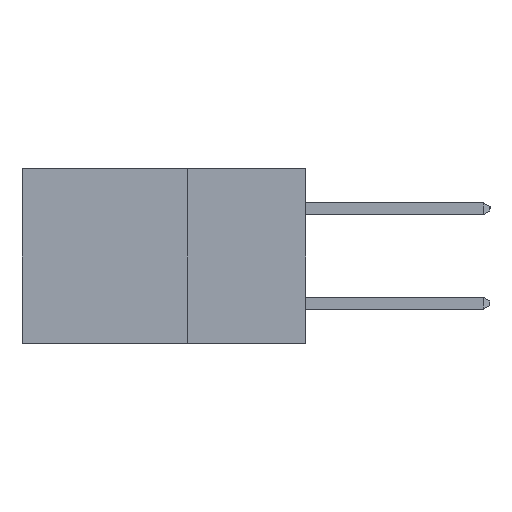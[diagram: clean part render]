
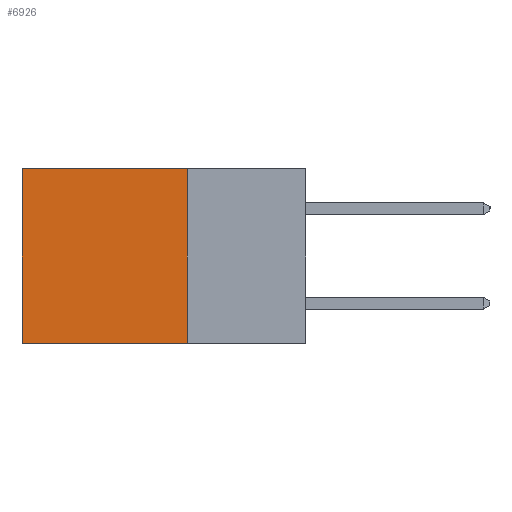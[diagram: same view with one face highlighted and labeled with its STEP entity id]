
A CAD part, left-side view. The second image highlights one B-rep face of the part: STEP entity #6926.
In plain terms, the highlighted planar face has unit normal (-1, 0, 0).
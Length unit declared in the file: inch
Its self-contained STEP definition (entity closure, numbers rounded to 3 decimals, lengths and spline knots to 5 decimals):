
#310 = EDGE_LOOP ( 'NONE', ( #14567, #15046, #4161, #5127 ) ) ;
#1045 = CARTESIAN_POINT ( 'NONE',  ( 0.2615, 0.25, -0.37 ) ) ;
#1095 = VECTOR ( 'NONE', #6059, 39.37008 ) ;
#2472 = LINE ( 'NONE', #10881, #1095 ) ;
#2855 = DIRECTION ( 'NONE',  ( 0., 0., -1. ) ) ;
#3268 = EDGE_CURVE ( 'NONE', #10681, #4784, #2472, .T. ) ;
#3337 = CARTESIAN_POINT ( 'NONE',  ( 0.2615, 0.25, 0. ) ) ;
#4161 = ORIENTED_EDGE ( 'NONE', *, *, #4884, .F. ) ;
#4784 = VERTEX_POINT ( 'NONE', #5743 ) ;
#4786 = EDGE_CURVE ( 'NONE', #7679, #4784, #14224, .T. ) ;
#4884 = EDGE_CURVE ( 'NONE', #8909, #10681, #15176, .T. ) ;
#5127 = ORIENTED_EDGE ( 'NONE', *, *, #6006, .T. ) ;
#5743 = CARTESIAN_POINT ( 'NONE',  ( 0.2615, 0.6, -0.37 ) ) ;
#6006 = EDGE_CURVE ( 'NONE', #8909, #7679, #7946, .T. ) ;
#6059 = DIRECTION ( 'NONE',  ( 0., 1., 0. ) ) ;
#6742 = CARTESIAN_POINT ( 'NONE',  ( 0.2615, 0.6, 0. ) ) ;
#6861 = VECTOR ( 'NONE', #9268, 39.37008 ) ;
#6926 = ADVANCED_FACE ( 'NONE', ( #14705 ), #13610, .F. ) ;
#6980 = CARTESIAN_POINT ( 'NONE',  ( 0.2615, 0.25, 0. ) ) ;
#7623 = AXIS2_PLACEMENT_3D ( 'NONE', #8775, #10089, #2855 ) ;
#7679 = VERTEX_POINT ( 'NONE', #6742 ) ;
#7946 = LINE ( 'NONE', #3337, #6861 ) ;
#8065 = CARTESIAN_POINT ( 'NONE',  ( 0.2615, 0.6, -0.37 ) ) ;
#8566 = VECTOR ( 'NONE', #12982, 39.37008 ) ;
#8775 = CARTESIAN_POINT ( 'NONE',  ( 0.2615, 0.25, -0.37 ) ) ;
#8909 = VERTEX_POINT ( 'NONE', #6980 ) ;
#9246 = DIRECTION ( 'NONE',  ( 0., 0., -1. ) ) ;
#9268 = DIRECTION ( 'NONE',  ( 0., 1., 0. ) ) ;
#10089 = DIRECTION ( 'NONE',  ( 1., 0., 0. ) ) ;
#10681 = VERTEX_POINT ( 'NONE', #11320 ) ;
#10881 = CARTESIAN_POINT ( 'NONE',  ( 0.2615, 0.25, -0.37 ) ) ;
#11320 = CARTESIAN_POINT ( 'NONE',  ( 0.2615, 0.25, -0.37 ) ) ;
#12306 = VECTOR ( 'NONE', #9246, 39.37008 ) ;
#12982 = DIRECTION ( 'NONE',  ( 0., 0., -1. ) ) ;
#13610 = PLANE ( 'NONE',  #7623 ) ;
#14224 = LINE ( 'NONE', #8065, #8566 ) ;
#14567 = ORIENTED_EDGE ( 'NONE', *, *, #4786, .T. ) ;
#14705 = FACE_OUTER_BOUND ( 'NONE', #310, .T. ) ;
#15046 = ORIENTED_EDGE ( 'NONE', *, *, #3268, .F. ) ;
#15176 = LINE ( 'NONE', #1045, #12306 ) ;
